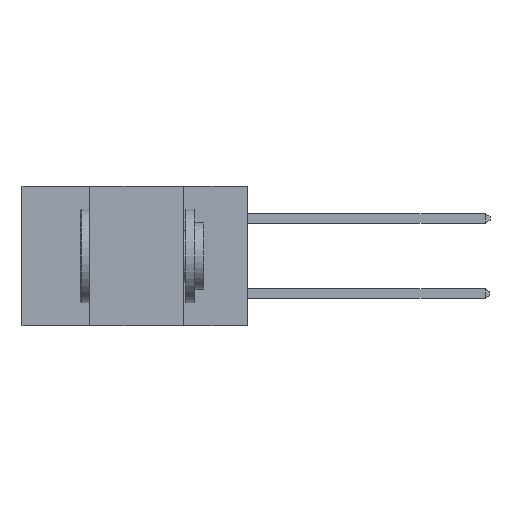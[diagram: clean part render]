
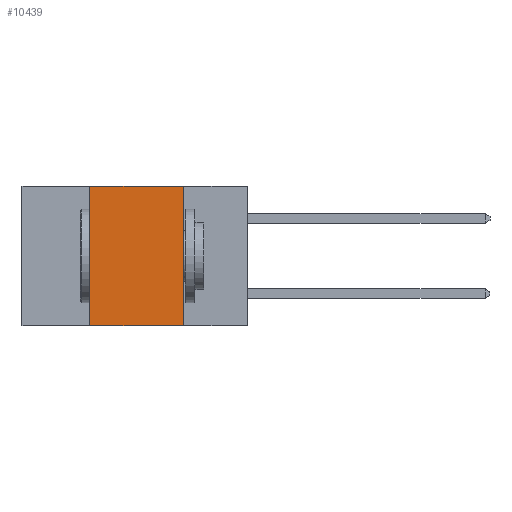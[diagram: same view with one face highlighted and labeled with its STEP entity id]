
A CAD part, left-side view. The second image highlights one B-rep face of the part: STEP entity #10439.
In plain terms, the highlighted planar face has unit normal (-1, 0, 0).
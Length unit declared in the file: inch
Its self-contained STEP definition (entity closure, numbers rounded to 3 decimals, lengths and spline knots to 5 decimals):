
#43 = LINE ( 'NONE', #7700, #2989 ) ;
#1668 = LINE ( 'NONE', #11161, #4218 ) ;
#1976 = AXIS2_PLACEMENT_3D ( 'NONE', #5831, #14464, #7115 ) ;
#2155 = EDGE_CURVE ( 'NONE', #6037, #4673, #43, .T. ) ;
#2564 = DIRECTION ( 'NONE',  ( 0., 0., 1. ) ) ;
#2989 = VECTOR ( 'NONE', #8321, 39.37008 ) ;
#3374 = VERTEX_POINT ( 'NONE', #15414 ) ;
#3547 = DIRECTION ( 'NONE',  ( 0., 0., -1. ) ) ;
#4070 = EDGE_CURVE ( 'NONE', #6037, #3374, #4702, .T. ) ;
#4218 = VECTOR ( 'NONE', #3547, 39.37008 ) ;
#4230 = CARTESIAN_POINT ( 'NONE',  ( 0., 0.17, 0. ) ) ;
#4409 = DIRECTION ( 'NONE',  ( 0., -1., 0. ) ) ;
#4673 = VERTEX_POINT ( 'NONE', #5946 ) ;
#4702 = LINE ( 'NONE', #9225, #14186 ) ;
#5831 = CARTESIAN_POINT ( 'NONE',  ( 0., 0.6, 0. ) ) ;
#5946 = CARTESIAN_POINT ( 'NONE',  ( 0., 0.17, -0.37 ) ) ;
#6037 = VERTEX_POINT ( 'NONE', #15820 ) ;
#6973 = ORIENTED_EDGE ( 'NONE', *, *, #13821, .F. ) ;
#7115 = DIRECTION ( 'NONE',  ( 0., 0., -1. ) ) ;
#7225 = EDGE_CURVE ( 'NONE', #11643, #4673, #1668, .T. ) ;
#7621 = EDGE_LOOP ( 'NONE', ( #9064, #6973, #15938, #11206 ) ) ;
#7700 = CARTESIAN_POINT ( 'NONE',  ( 0., 0.6, -0.37 ) ) ;
#8160 = CARTESIAN_POINT ( 'NONE',  ( 0., 0.6, 0. ) ) ;
#8245 = VECTOR ( 'NONE', #4409, 39.37008 ) ;
#8321 = DIRECTION ( 'NONE',  ( 0., -1., 0. ) ) ;
#9064 = ORIENTED_EDGE ( 'NONE', *, *, #7225, .F. ) ;
#9225 = CARTESIAN_POINT ( 'NONE',  ( 0., 0.42, 0. ) ) ;
#10439 = ADVANCED_FACE ( 'NONE', ( #12538 ), #10883, .F. ) ;
#10883 = PLANE ( 'NONE',  #1976 ) ;
#11161 = CARTESIAN_POINT ( 'NONE',  ( 0., 0.17, 0. ) ) ;
#11206 = ORIENTED_EDGE ( 'NONE', *, *, #2155, .T. ) ;
#11643 = VERTEX_POINT ( 'NONE', #4230 ) ;
#12538 = FACE_OUTER_BOUND ( 'NONE', #7621, .T. ) ;
#13821 = EDGE_CURVE ( 'NONE', #3374, #11643, #13928, .T. ) ;
#13928 = LINE ( 'NONE', #8160, #8245 ) ;
#14186 = VECTOR ( 'NONE', #2564, 39.37008 ) ;
#14464 = DIRECTION ( 'NONE',  ( 1., 0., 0. ) ) ;
#15414 = CARTESIAN_POINT ( 'NONE',  ( 0., 0.42, 0. ) ) ;
#15820 = CARTESIAN_POINT ( 'NONE',  ( 0., 0.42, -0.37 ) ) ;
#15938 = ORIENTED_EDGE ( 'NONE', *, *, #4070, .F. ) ;
